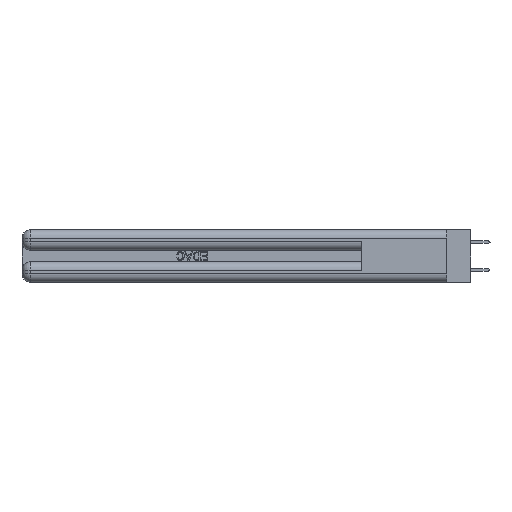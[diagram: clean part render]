
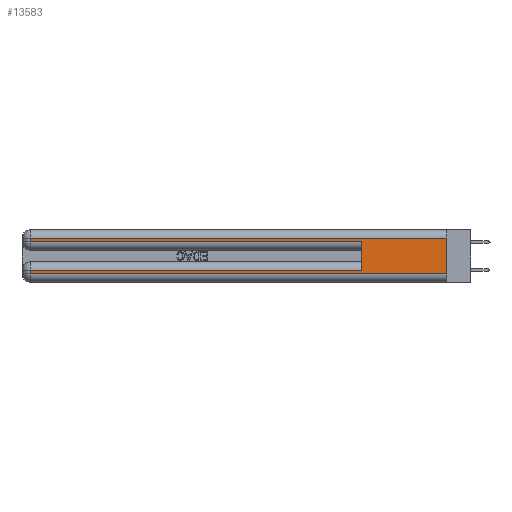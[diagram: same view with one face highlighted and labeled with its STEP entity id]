
A CAD part, left-side view. The second image highlights one B-rep face of the part: STEP entity #13583.
In plain terms, the highlighted planar face has unit normal (-1, 0, 0).
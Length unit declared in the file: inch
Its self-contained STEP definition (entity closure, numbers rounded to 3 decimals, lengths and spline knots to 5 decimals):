
#316 = CARTESIAN_POINT ( 'NONE',  ( 0., 0., 0.085 ) ) ;
#2412 = LINE ( 'NONE', #49247, #50572 ) ;
#2641 = VECTOR ( 'NONE', #30947, 39.37008 ) ;
#3488 = VERTEX_POINT ( 'NONE', #27879 ) ;
#5232 = EDGE_CURVE ( 'NONE', #35172, #36420, #42698, .T. ) ;
#5325 = VERTEX_POINT ( 'NONE', #40755 ) ;
#6184 = CARTESIAN_POINT ( 'NONE',  ( 0., 0., 0.37 ) ) ;
#6420 = DIRECTION ( 'NONE',  ( 0., -1., 0. ) ) ;
#6442 = FACE_OUTER_BOUND ( 'NONE', #14212, .T. ) ;
#7051 = CARTESIAN_POINT ( 'NONE',  ( 0., 2.94, 0.085 ) ) ;
#10301 = LINE ( 'NONE', #26097, #50592 ) ;
#10628 = DIRECTION ( 'NONE',  ( 0., 0., -1. ) ) ;
#13583 = ADVANCED_FACE ( 'NONE', ( #6442 ), #21492, .F. ) ;
#14212 = EDGE_LOOP ( 'NONE', ( #18071, #29446, #22750, #48485, #48491, #29451, #35238, #40908 ) ) ;
#15120 = LINE ( 'NONE', #23406, #2641 ) ;
#16144 = DIRECTION ( 'NONE',  ( 0., 1., 0. ) ) ;
#18071 = ORIENTED_EDGE ( 'NONE', *, *, #21264, .F. ) ;
#18087 = LINE ( 'NONE', #33705, #35675 ) ;
#18246 = DIRECTION ( 'NONE',  ( 0., 0., -1. ) ) ;
#19418 = VECTOR ( 'NONE', #50519, 39.37008 ) ;
#19909 = VERTEX_POINT ( 'NONE', #25736 ) ;
#21264 = EDGE_CURVE ( 'NONE', #5325, #41103, #2412, .T. ) ;
#21492 = PLANE ( 'NONE',  #40968 ) ;
#21755 = VECTOR ( 'NONE', #10628, 39.37008 ) ;
#22750 = ORIENTED_EDGE ( 'NONE', *, *, #32376, .T. ) ;
#23406 = CARTESIAN_POINT ( 'NONE',  ( 0., 0., 0.285 ) ) ;
#24654 = CARTESIAN_POINT ( 'NONE',  ( 0., 0.6, 0.085 ) ) ;
#25736 = CARTESIAN_POINT ( 'NONE',  ( 0., 2.94, 0.31 ) ) ;
#26097 = CARTESIAN_POINT ( 'NONE',  ( 0., 0., 0.06 ) ) ;
#26107 = DIRECTION ( 'NONE',  ( 0., 0., -1. ) ) ;
#26175 = CARTESIAN_POINT ( 'NONE',  ( 0., 2.94, 0.37 ) ) ;
#27861 = CARTESIAN_POINT ( 'NONE',  ( 0., 0., 0.06 ) ) ;
#27879 = CARTESIAN_POINT ( 'NONE',  ( 0., 2.94, 0.285 ) ) ;
#28080 = EDGE_CURVE ( 'NONE', #30242, #41103, #10301, .T. ) ;
#28736 = EDGE_CURVE ( 'NONE', #5325, #19909, #44048, .T. ) ;
#29306 = EDGE_CURVE ( 'NONE', #37885, #30242, #18087, .T. ) ;
#29446 = ORIENTED_EDGE ( 'NONE', *, *, #28736, .T. ) ;
#29451 = ORIENTED_EDGE ( 'NONE', *, *, #50521, .T. ) ;
#30064 = DIRECTION ( 'NONE',  ( 1., 0., 0. ) ) ;
#30242 = VERTEX_POINT ( 'NONE', #43006 ) ;
#30947 = DIRECTION ( 'NONE',  ( 0., -1., 0. ) ) ;
#32376 = EDGE_CURVE ( 'NONE', #19909, #3488, #45754, .T. ) ;
#33352 = EDGE_CURVE ( 'NONE', #3488, #36420, #15120, .T. ) ;
#33705 = CARTESIAN_POINT ( 'NONE',  ( 0., 2.94, 0.37 ) ) ;
#33717 = DIRECTION ( 'NONE',  ( 0., 0., -1. ) ) ;
#35172 = VERTEX_POINT ( 'NONE', #24654 ) ;
#35238 = ORIENTED_EDGE ( 'NONE', *, *, #29306, .T. ) ;
#35675 = VECTOR ( 'NONE', #26107, 39.37008 ) ;
#35676 = CARTESIAN_POINT ( 'NONE',  ( 0., 0.6, 0.285 ) ) ;
#35887 = LINE ( 'NONE', #316, #45027 ) ;
#36420 = VERTEX_POINT ( 'NONE', #35676 ) ;
#37885 = VERTEX_POINT ( 'NONE', #7051 ) ;
#38253 = CARTESIAN_POINT ( 'NONE',  ( 0., 0.6, 0.145 ) ) ;
#40367 = CARTESIAN_POINT ( 'NONE',  ( 0., 0., 0.31 ) ) ;
#40755 = CARTESIAN_POINT ( 'NONE',  ( 0., 0., 0.31 ) ) ;
#40908 = ORIENTED_EDGE ( 'NONE', *, *, #28080, .T. ) ;
#40968 = AXIS2_PLACEMENT_3D ( 'NONE', #6184, #30064, #33717 ) ;
#41103 = VERTEX_POINT ( 'NONE', #27861 ) ;
#42698 = LINE ( 'NONE', #38253, #19418 ) ;
#43006 = CARTESIAN_POINT ( 'NONE',  ( 0., 2.94, 0.06 ) ) ;
#44048 = LINE ( 'NONE', #40367, #44802 ) ;
#44539 = DIRECTION ( 'NONE',  ( 0., 1., 0. ) ) ;
#44802 = VECTOR ( 'NONE', #44539, 39.37008 ) ;
#45027 = VECTOR ( 'NONE', #16144, 39.37008 ) ;
#45754 = LINE ( 'NONE', #26175, #21755 ) ;
#48485 = ORIENTED_EDGE ( 'NONE', *, *, #33352, .T. ) ;
#48491 = ORIENTED_EDGE ( 'NONE', *, *, #5232, .F. ) ;
#49247 = CARTESIAN_POINT ( 'NONE',  ( 0., 0., 0.37 ) ) ;
#50519 = DIRECTION ( 'NONE',  ( 0., 0., 1. ) ) ;
#50521 = EDGE_CURVE ( 'NONE', #35172, #37885, #35887, .T. ) ;
#50572 = VECTOR ( 'NONE', #18246, 39.37008 ) ;
#50592 = VECTOR ( 'NONE', #6420, 39.37008 ) ;
